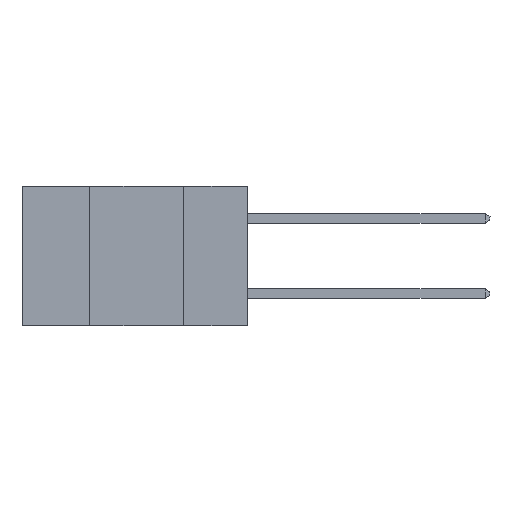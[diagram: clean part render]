
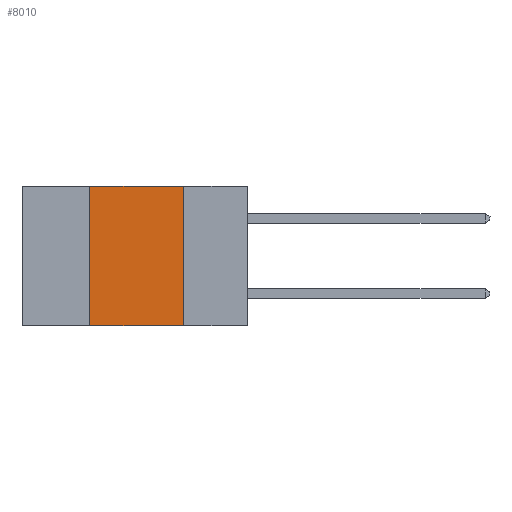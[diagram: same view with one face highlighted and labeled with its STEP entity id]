
A CAD part, left-side view. The second image highlights one B-rep face of the part: STEP entity #8010.
In plain terms, the highlighted planar face has unit normal (-1, 0, 0).
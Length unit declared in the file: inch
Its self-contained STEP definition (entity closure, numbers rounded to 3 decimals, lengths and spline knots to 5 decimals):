
#211 = EDGE_CURVE ( 'NONE', #1260, #4709, #9078, .T. ) ;
#432 = EDGE_CURVE ( 'NONE', #4709, #5218, #3278, .T. ) ;
#1079 = CARTESIAN_POINT ( 'NONE',  ( 0., 0.6, -0.37 ) ) ;
#1239 = CARTESIAN_POINT ( 'NONE',  ( 0., 0.17, -0.37 ) ) ;
#1260 = VERTEX_POINT ( 'NONE', #8124 ) ;
#1292 = DIRECTION ( 'NONE',  ( 1., 0., 0. ) ) ;
#1439 = LINE ( 'NONE', #4626, #3573 ) ;
#1758 = ORIENTED_EDGE ( 'NONE', *, *, #211, .F. ) ;
#2077 = FACE_OUTER_BOUND ( 'NONE', #3347, .T. ) ;
#2617 = CARTESIAN_POINT ( 'NONE',  ( 0., 0.6, 0. ) ) ;
#2772 = DIRECTION ( 'NONE',  ( 0., 0., -1. ) ) ;
#3278 = LINE ( 'NONE', #2617, #5007 ) ;
#3347 = EDGE_LOOP ( 'NONE', ( #5599, #8277, #1758, #5659 ) ) ;
#3567 = PLANE ( 'NONE',  #4646 ) ;
#3573 = VECTOR ( 'NONE', #3869, 39.37008 ) ;
#3869 = DIRECTION ( 'NONE',  ( 0., 0., -1. ) ) ;
#4039 = DIRECTION ( 'NONE',  ( 0., 0., 1. ) ) ;
#4133 = EDGE_CURVE ( 'NONE', #1260, #4392, #5802, .T. ) ;
#4392 = VERTEX_POINT ( 'NONE', #1239 ) ;
#4626 = CARTESIAN_POINT ( 'NONE',  ( 0., 0.17, -0.37 ) ) ;
#4646 = AXIS2_PLACEMENT_3D ( 'NONE', #6689, #1292, #2772 ) ;
#4709 = VERTEX_POINT ( 'NONE', #4932 ) ;
#4932 = CARTESIAN_POINT ( 'NONE',  ( 0., 0.42, 0. ) ) ;
#5007 = VECTOR ( 'NONE', #7213, 39.37008 ) ;
#5218 = VERTEX_POINT ( 'NONE', #6833 ) ;
#5599 = ORIENTED_EDGE ( 'NONE', *, *, #9327, .F. ) ;
#5659 = ORIENTED_EDGE ( 'NONE', *, *, #4133, .T. ) ;
#5802 = LINE ( 'NONE', #1079, #8578 ) ;
#6635 = VECTOR ( 'NONE', #4039, 39.37008 ) ;
#6689 = CARTESIAN_POINT ( 'NONE',  ( 0., 0.6, 0. ) ) ;
#6833 = CARTESIAN_POINT ( 'NONE',  ( 0., 0.17, 0. ) ) ;
#7213 = DIRECTION ( 'NONE',  ( 0., -1., 0. ) ) ;
#8010 = ADVANCED_FACE ( 'NONE', ( #2077 ), #3567, .F. ) ;
#8124 = CARTESIAN_POINT ( 'NONE',  ( 0., 0.42, -0.37 ) ) ;
#8277 = ORIENTED_EDGE ( 'NONE', *, *, #432, .F. ) ;
#8578 = VECTOR ( 'NONE', #9825, 39.37008 ) ;
#9078 = LINE ( 'NONE', #9450, #6635 ) ;
#9327 = EDGE_CURVE ( 'NONE', #5218, #4392, #1439, .T. ) ;
#9450 = CARTESIAN_POINT ( 'NONE',  ( 0., 0.42, -0.37 ) ) ;
#9825 = DIRECTION ( 'NONE',  ( 0., -1., 0. ) ) ;
